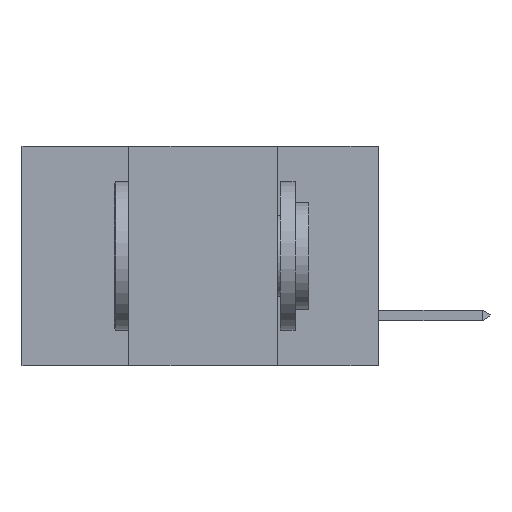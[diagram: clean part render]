
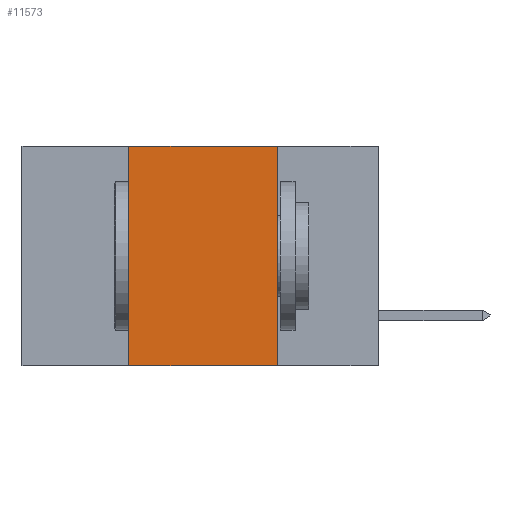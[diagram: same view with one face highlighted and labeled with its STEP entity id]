
A CAD part, left-side view. The second image highlights one B-rep face of the part: STEP entity #11573.
In plain terms, the highlighted planar face has unit normal (-1, 0, 0).
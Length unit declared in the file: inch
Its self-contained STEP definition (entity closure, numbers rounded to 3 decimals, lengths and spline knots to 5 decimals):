
#418 = DIRECTION ( 'NONE',  ( 0., -1., 0. ) ) ;
#419 = CARTESIAN_POINT ( 'NONE',  ( 0., 0.42, 0. ) ) ;
#585 = VECTOR ( 'NONE', #418, 39.37008 ) ;
#1201 = DIRECTION ( 'NONE',  ( 0., 0., 1. ) ) ;
#1257 = CARTESIAN_POINT ( 'NONE',  ( 0., 0.42, 0. ) ) ;
#2430 = EDGE_LOOP ( 'NONE', ( #11865, #12179, #5102, #4913 ) ) ;
#2745 = VECTOR ( 'NONE', #9276, 39.37008 ) ;
#2780 = EDGE_CURVE ( 'NONE', #10771, #8747, #6731, .T. ) ;
#2938 = VECTOR ( 'NONE', #1201, 39.37008 ) ;
#3175 = DIRECTION ( 'NONE',  ( 1., 0., 0. ) ) ;
#4025 = LINE ( 'NONE', #13424, #2745 ) ;
#4913 = ORIENTED_EDGE ( 'NONE', *, *, #14922, .T. ) ;
#5102 = ORIENTED_EDGE ( 'NONE', *, *, #2780, .F. ) ;
#5256 = CARTESIAN_POINT ( 'NONE',  ( 0., 0.17, 0. ) ) ;
#5734 = CARTESIAN_POINT ( 'NONE',  ( 0., 0.6, 0. ) ) ;
#5775 = CARTESIAN_POINT ( 'NONE',  ( 0., 0.6, 0. ) ) ;
#6105 = CARTESIAN_POINT ( 'NONE',  ( 0., 0.42, -0.37 ) ) ;
#6331 = CARTESIAN_POINT ( 'NONE',  ( 0., 0.17, -0.37 ) ) ;
#6731 = LINE ( 'NONE', #1257, #2938 ) ;
#7196 = DIRECTION ( 'NONE',  ( 0., 0., -1. ) ) ;
#7768 = LINE ( 'NONE', #5734, #585 ) ;
#8196 = FACE_OUTER_BOUND ( 'NONE', #2430, .T. ) ;
#8747 = VERTEX_POINT ( 'NONE', #419 ) ;
#9276 = DIRECTION ( 'NONE',  ( 0., 0., -1. ) ) ;
#10771 = VERTEX_POINT ( 'NONE', #6105 ) ;
#10899 = DIRECTION ( 'NONE',  ( 0., -1., 0. ) ) ;
#11573 = ADVANCED_FACE ( 'NONE', ( #8196 ), #14035, .F. ) ;
#11687 = VECTOR ( 'NONE', #10899, 39.37008 ) ;
#11865 = ORIENTED_EDGE ( 'NONE', *, *, #17385, .F. ) ;
#11976 = EDGE_CURVE ( 'NONE', #8747, #13688, #7768, .T. ) ;
#12179 = ORIENTED_EDGE ( 'NONE', *, *, #11976, .F. ) ;
#13424 = CARTESIAN_POINT ( 'NONE',  ( 0., 0.17, 0. ) ) ;
#13607 = AXIS2_PLACEMENT_3D ( 'NONE', #5775, #3175, #7196 ) ;
#13688 = VERTEX_POINT ( 'NONE', #5256 ) ;
#14035 = PLANE ( 'NONE',  #13607 ) ;
#14308 = VERTEX_POINT ( 'NONE', #6331 ) ;
#14922 = EDGE_CURVE ( 'NONE', #10771, #14308, #15219, .T. ) ;
#15219 = LINE ( 'NONE', #16268, #11687 ) ;
#16268 = CARTESIAN_POINT ( 'NONE',  ( 0., 0.6, -0.37 ) ) ;
#17385 = EDGE_CURVE ( 'NONE', #13688, #14308, #4025, .T. ) ;
